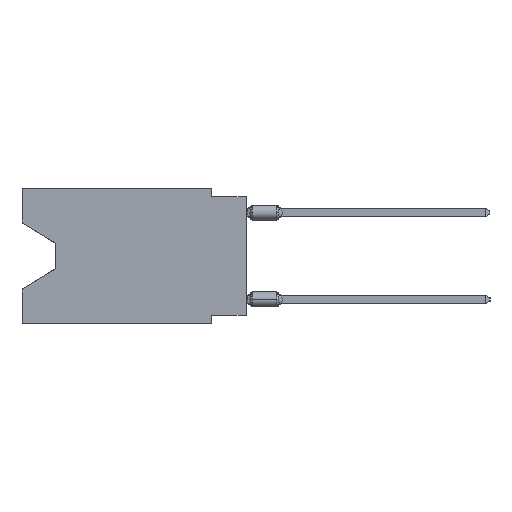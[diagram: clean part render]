
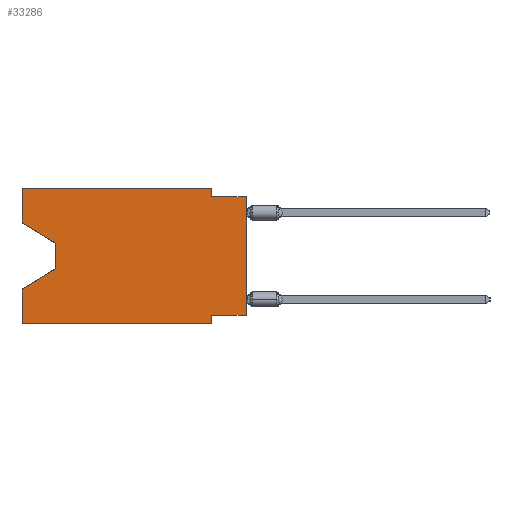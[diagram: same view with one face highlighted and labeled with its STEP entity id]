
A CAD part, left-side view. The second image highlights one B-rep face of the part: STEP entity #33286.
In plain terms, the highlighted planar face has unit normal (-1, 0, 0).
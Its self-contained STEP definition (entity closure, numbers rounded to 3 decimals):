
#103 = EDGE_CURVE ( 'NONE', #9923, #59017, #3608, .T. ) ;
#332 = LINE ( 'NONE', #62645, #44556 ) ;
#396 = VECTOR ( 'NONE', #12524, 1000. ) ;
#1369 = CARTESIAN_POINT ( 'NONE',  ( 0., 0., -9.271 ) ) ;
#1435 = CARTESIAN_POINT ( 'NONE',  ( 0., 16.383, -2.546 ) ) ;
#2081 = LINE ( 'NONE', #16513, #19539 ) ;
#2168 = LINE ( 'NONE', #48399, #12174 ) ;
#3608 = LINE ( 'NONE', #49188, #49181 ) ;
#4051 = LINE ( 'NONE', #24510, #48569 ) ;
#6189 = VERTEX_POINT ( 'NONE', #1369 ) ;
#7121 = DIRECTION ( 'NONE',  ( 0., -1., 0. ) ) ;
#7451 = LINE ( 'NONE', #32916, #10022 ) ;
#7632 = PLANE ( 'NONE',  #16395 ) ;
#9100 = CARTESIAN_POINT ( 'NONE',  ( 0., 13.97, -5.893 ) ) ;
#9153 = VERTEX_POINT ( 'NONE', #17488 ) ;
#9923 = VERTEX_POINT ( 'NONE', #60889 ) ;
#10022 = VECTOR ( 'NONE', #7121, 1000. ) ;
#10831 = CARTESIAN_POINT ( 'NONE',  ( 0., 2.54, -0.635 ) ) ;
#11084 = ORIENTED_EDGE ( 'NONE', *, *, #38334, .T. ) ;
#12174 = VECTOR ( 'NONE', #58139, 1000. ) ;
#12230 = CARTESIAN_POINT ( 'NONE',  ( 0., 16.383, -9.906 ) ) ;
#12524 = DIRECTION ( 'NONE',  ( 0., 0., -1. ) ) ;
#14057 = DIRECTION ( 'NONE',  ( 0., 0., 1. ) ) ;
#16240 = VECTOR ( 'NONE', #14057, 1000. ) ;
#16395 = AXIS2_PLACEMENT_3D ( 'NONE', #43156, #48514, #17709 ) ;
#16513 = CARTESIAN_POINT ( 'NONE',  ( 0., 13.97, -5.893 ) ) ;
#17488 = CARTESIAN_POINT ( 'NONE',  ( 0., 2.54, -9.271 ) ) ;
#17507 = EDGE_CURVE ( 'NONE', #39815, #59017, #2081, .T. ) ;
#17709 = DIRECTION ( 'NONE',  ( 0., 0., -1. ) ) ;
#18692 = VERTEX_POINT ( 'NONE', #22835 ) ;
#18749 = ORIENTED_EDGE ( 'NONE', *, *, #103, .F. ) ;
#19247 = VERTEX_POINT ( 'NONE', #19365 ) ;
#19365 = CARTESIAN_POINT ( 'NONE',  ( 0., 2.54, -9.906 ) ) ;
#19539 = VECTOR ( 'NONE', #42622, 1000. ) ;
#21944 = CARTESIAN_POINT ( 'NONE',  ( 0., 2.54, 0. ) ) ;
#22403 = DIRECTION ( 'NONE',  ( 0., -1., 0. ) ) ;
#22835 = CARTESIAN_POINT ( 'NONE',  ( 0., 16.383, 0. ) ) ;
#24510 = CARTESIAN_POINT ( 'NONE',  ( 0., 13.97, -4.013 ) ) ;
#25167 = DIRECTION ( 'NONE',  ( 0., 0., -1. ) ) ;
#27651 = DIRECTION ( 'NONE',  ( 0., -1., 0. ) ) ;
#27760 = FACE_OUTER_BOUND ( 'NONE', #60513, .T. ) ;
#28758 = DIRECTION ( 'NONE',  ( 0., 0., 1. ) ) ;
#29162 = VECTOR ( 'NONE', #27651, 1000. ) ;
#30804 = EDGE_CURVE ( 'NONE', #9923, #19247, #58150, .T. ) ;
#31571 = ORIENTED_EDGE ( 'NONE', *, *, #33904, .F. ) ;
#31648 = LINE ( 'NONE', #21944, #396 ) ;
#31812 = EDGE_CURVE ( 'NONE', #6189, #59982, #64980, .T. ) ;
#31971 = DIRECTION ( 'NONE',  ( 0., 1., 0. ) ) ;
#32033 = EDGE_CURVE ( 'NONE', #35600, #59982, #58560, .T. ) ;
#32428 = ORIENTED_EDGE ( 'NONE', *, *, #66237, .F. ) ;
#32441 = CARTESIAN_POINT ( 'NONE',  ( 0., 0., -0.635 ) ) ;
#32916 = CARTESIAN_POINT ( 'NONE',  ( 0., 16.383, 0. ) ) ;
#32951 = VERTEX_POINT ( 'NONE', #35143 ) ;
#33286 = ADVANCED_FACE ( 'NONE', ( #27760 ), #7632, .F. ) ;
#33396 = VECTOR ( 'NONE', #22403, 1000. ) ;
#33904 = EDGE_CURVE ( 'NONE', #18692, #45006, #7451, .T. ) ;
#35143 = CARTESIAN_POINT ( 'NONE',  ( 0., 13.97, -4.013 ) ) ;
#35600 = VERTEX_POINT ( 'NONE', #10831 ) ;
#38334 = EDGE_CURVE ( 'NONE', #56921, #32951, #41635, .T. ) ;
#38843 = ORIENTED_EDGE ( 'NONE', *, *, #51060, .F. ) ;
#39512 = CARTESIAN_POINT ( 'NONE',  ( 0., 0., 0. ) ) ;
#39815 = VERTEX_POINT ( 'NONE', #9100 ) ;
#41635 = LINE ( 'NONE', #1435, #58406 ) ;
#41967 = DIRECTION ( 'NONE',  ( 0., -0.855, -0.519 ) ) ;
#42358 = VECTOR ( 'NONE', #31971, 1000. ) ;
#42622 = DIRECTION ( 'NONE',  ( 0., 0.855, -0.519 ) ) ;
#43156 = CARTESIAN_POINT ( 'NONE',  ( 0., 16.383, 0. ) ) ;
#43633 = ORIENTED_EDGE ( 'NONE', *, *, #50218, .F. ) ;
#43991 = ORIENTED_EDGE ( 'NONE', *, *, #32033, .F. ) ;
#44556 = VECTOR ( 'NONE', #46560, 1000. ) ;
#45006 = VERTEX_POINT ( 'NONE', #53449 ) ;
#45300 = CARTESIAN_POINT ( 'NONE',  ( 0., 0., -0.635 ) ) ;
#45548 = ORIENTED_EDGE ( 'NONE', *, *, #46371, .F. ) ;
#46371 = EDGE_CURVE ( 'NONE', #45006, #35600, #31648, .T. ) ;
#46560 = DIRECTION ( 'NONE',  ( 0., 0., -1. ) ) ;
#47674 = CARTESIAN_POINT ( 'NONE',  ( 0., 16.383, -2.546 ) ) ;
#48394 = EDGE_CURVE ( 'NONE', #32951, #39815, #4051, .T. ) ;
#48399 = CARTESIAN_POINT ( 'NONE',  ( 0., 16.383, 0. ) ) ;
#48514 = DIRECTION ( 'NONE',  ( 1., 0., 0. ) ) ;
#48569 = VECTOR ( 'NONE', #25167, 1000. ) ;
#49181 = VECTOR ( 'NONE', #28758, 1000. ) ;
#49188 = CARTESIAN_POINT ( 'NONE',  ( 0., 16.383, 0. ) ) ;
#50218 = EDGE_CURVE ( 'NONE', #6189, #9153, #62133, .T. ) ;
#51060 = EDGE_CURVE ( 'NONE', #9153, #19247, #332, .T. ) ;
#53449 = CARTESIAN_POINT ( 'NONE',  ( 0., 2.54, 0. ) ) ;
#54529 = CARTESIAN_POINT ( 'NONE',  ( 0., 16.383, -7.36 ) ) ;
#54703 = ORIENTED_EDGE ( 'NONE', *, *, #31812, .T. ) ;
#54903 = ORIENTED_EDGE ( 'NONE', *, *, #48394, .T. ) ;
#56921 = VERTEX_POINT ( 'NONE', #47674 ) ;
#58139 = DIRECTION ( 'NONE',  ( 0., 0., 1. ) ) ;
#58150 = LINE ( 'NONE', #12230, #29162 ) ;
#58406 = VECTOR ( 'NONE', #41967, 1000. ) ;
#58560 = LINE ( 'NONE', #32441, #33396 ) ;
#59017 = VERTEX_POINT ( 'NONE', #54529 ) ;
#59969 = ORIENTED_EDGE ( 'NONE', *, *, #17507, .T. ) ;
#59982 = VERTEX_POINT ( 'NONE', #45300 ) ;
#60513 = EDGE_LOOP ( 'NONE', ( #11084, #54903, #59969, #18749, #64150, #38843, #43633, #54703, #43991, #45548, #31571, #32428 ) ) ;
#60889 = CARTESIAN_POINT ( 'NONE',  ( 0., 16.383, -9.906 ) ) ;
#61790 = CARTESIAN_POINT ( 'NONE',  ( 0., 0., -9.271 ) ) ;
#62133 = LINE ( 'NONE', #61790, #42358 ) ;
#62645 = CARTESIAN_POINT ( 'NONE',  ( 0., 2.54, -9.906 ) ) ;
#64150 = ORIENTED_EDGE ( 'NONE', *, *, #30804, .T. ) ;
#64980 = LINE ( 'NONE', #39512, #16240 ) ;
#66237 = EDGE_CURVE ( 'NONE', #56921, #18692, #2168, .T. ) ;
